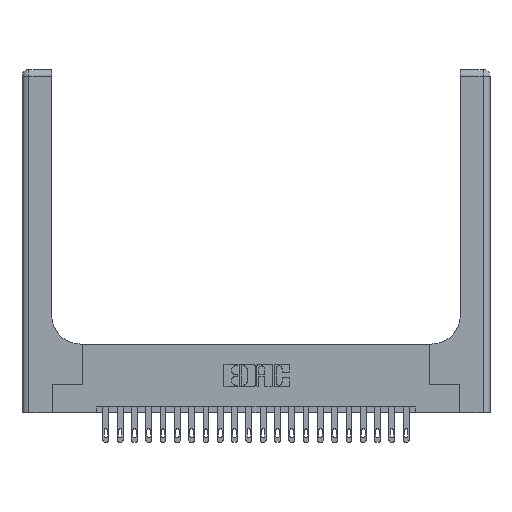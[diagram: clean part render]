
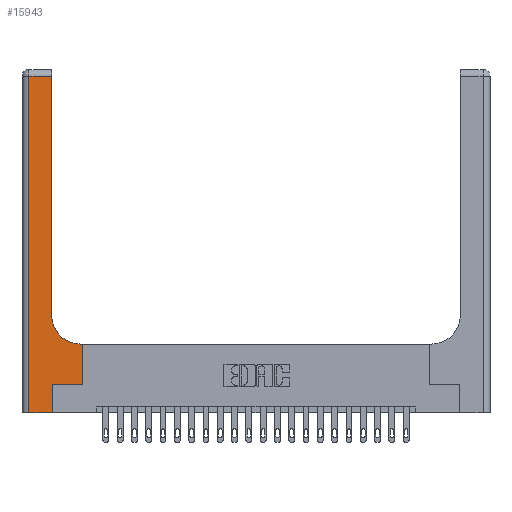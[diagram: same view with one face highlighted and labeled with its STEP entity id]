
A CAD part, top view. The second image highlights one B-rep face of the part: STEP entity #15943.
In plain terms, the highlighted planar face has unit normal (0, 0, 1).
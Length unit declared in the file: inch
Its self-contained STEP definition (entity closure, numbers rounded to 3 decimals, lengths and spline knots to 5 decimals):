
#837 = LINE ( 'NONE', #6121, #18668 ) ;
#1237 = LINE ( 'NONE', #21724, #15474 ) ;
#1333 = VERTEX_POINT ( 'NONE', #20239 ) ;
#1454 = CARTESIAN_POINT ( 'NONE',  ( 0.51, 0.6, 0.37 ) ) ;
#1460 = ORIENTED_EDGE ( 'NONE', *, *, #13298, .T. ) ;
#1658 = AXIS2_PLACEMENT_3D ( 'NONE', #1667, #21131, #7371 ) ;
#1667 = CARTESIAN_POINT ( 'NONE',  ( 0.51, 0.85, 0.37 ) ) ;
#2222 = LINE ( 'NONE', #19286, #21287 ) ;
#2387 = CARTESIAN_POINT ( 'NONE',  ( 0.06, 0., 0.37 ) ) ;
#2440 = DIRECTION ( 'NONE',  ( -1., 0., 0. ) ) ;
#2562 = DIRECTION ( 'NONE',  ( -1., 0., 0. ) ) ;
#3613 = DIRECTION ( 'NONE',  ( 0., 1., 0. ) ) ;
#3984 = ORIENTED_EDGE ( 'NONE', *, *, #19985, .T. ) ;
#4340 = EDGE_CURVE ( 'NONE', #7423, #19942, #9460, .T. ) ;
#4739 = EDGE_CURVE ( 'NONE', #1333, #20100, #837, .T. ) ;
#4877 = EDGE_CURVE ( 'NONE', #13815, #1333, #10093, .T. ) ;
#5120 = ORIENTED_EDGE ( 'NONE', *, *, #4877, .T. ) ;
#5781 = VECTOR ( 'NONE', #2562, 39.37008 ) ;
#6121 = CARTESIAN_POINT ( 'NONE',  ( 0.26, 0.6, 0.37 ) ) ;
#6176 = VERTEX_POINT ( 'NONE', #2387 ) ;
#6361 = ORIENTED_EDGE ( 'NONE', *, *, #13283, .T. ) ;
#6699 = CARTESIAN_POINT ( 'NONE',  ( 0.26, 2.94, 0.37 ) ) ;
#6926 = EDGE_CURVE ( 'NONE', #20100, #11942, #7878, .T. ) ;
#7192 = VERTEX_POINT ( 'NONE', #6699 ) ;
#7371 = DIRECTION ( 'NONE',  ( 1., 0., 0. ) ) ;
#7423 = VERTEX_POINT ( 'NONE', #18106 ) ;
#7878 = CIRCLE ( 'NONE', #1658, 0.25 ) ;
#8393 = VECTOR ( 'NONE', #16420, 39.37008 ) ;
#8433 = EDGE_LOOP ( 'NONE', ( #14188, #6361, #1460, #10906, #18893, #3984, #5120, #10993, #22576 ) ) ;
#9196 = AXIS2_PLACEMENT_3D ( 'NONE', #15601, #13441, #22366 ) ;
#9460 = LINE ( 'NONE', #11390, #8393 ) ;
#10093 = LINE ( 'NONE', #16956, #21581 ) ;
#10315 = DIRECTION ( 'NONE',  ( 0., 1., 0. ) ) ;
#10647 = EDGE_CURVE ( 'NONE', #6176, #7423, #16648, .T. ) ;
#10906 = ORIENTED_EDGE ( 'NONE', *, *, #10647, .T. ) ;
#10993 = ORIENTED_EDGE ( 'NONE', *, *, #4739, .T. ) ;
#11020 = LINE ( 'NONE', #16397, #12312 ) ;
#11390 = CARTESIAN_POINT ( 'NONE',  ( 0.265, 0., 0.37 ) ) ;
#11942 = VERTEX_POINT ( 'NONE', #13566 ) ;
#12312 = VECTOR ( 'NONE', #16170, 39.37008 ) ;
#12857 = CARTESIAN_POINT ( 'NONE',  ( 0., 0., 0.37 ) ) ;
#12948 = LINE ( 'NONE', #14680, #5781 ) ;
#13283 = EDGE_CURVE ( 'NONE', #7192, #22095, #12948, .T. ) ;
#13298 = EDGE_CURVE ( 'NONE', #22095, #6176, #11020, .T. ) ;
#13441 = DIRECTION ( 'NONE',  ( 0., 0., -1. ) ) ;
#13566 = CARTESIAN_POINT ( 'NONE',  ( 0.26, 0.85, 0.37 ) ) ;
#13815 = VERTEX_POINT ( 'NONE', #18553 ) ;
#14188 = ORIENTED_EDGE ( 'NONE', *, *, #16094, .T. ) ;
#14384 = CARTESIAN_POINT ( 'NONE',  ( 0.06, 2.94, 0.37 ) ) ;
#14680 = CARTESIAN_POINT ( 'NONE',  ( 0., 2.94, 0.37 ) ) ;
#15061 = DIRECTION ( 'NONE',  ( 1., 0., 0. ) ) ;
#15474 = VECTOR ( 'NONE', #15061, 39.37008 ) ;
#15601 = CARTESIAN_POINT ( 'NONE',  ( 0., 3., 0.37 ) ) ;
#15943 = ADVANCED_FACE ( 'NONE', ( #22256 ), #20567, .F. ) ;
#16094 = EDGE_CURVE ( 'NONE', #11942, #7192, #2222, .T. ) ;
#16170 = DIRECTION ( 'NONE',  ( 0., -1., 0. ) ) ;
#16397 = CARTESIAN_POINT ( 'NONE',  ( 0.06, 3., 0.37 ) ) ;
#16420 = DIRECTION ( 'NONE',  ( 0., 1., 0. ) ) ;
#16648 = LINE ( 'NONE', #12857, #17115 ) ;
#16956 = CARTESIAN_POINT ( 'NONE',  ( 0.528, 0.25, 0.37 ) ) ;
#17115 = VECTOR ( 'NONE', #18492, 39.37008 ) ;
#18106 = CARTESIAN_POINT ( 'NONE',  ( 0.265, 0., 0.37 ) ) ;
#18492 = DIRECTION ( 'NONE',  ( 1., 0., 0. ) ) ;
#18553 = CARTESIAN_POINT ( 'NONE',  ( 0.528, 0.25, 0.37 ) ) ;
#18668 = VECTOR ( 'NONE', #2440, 39.37008 ) ;
#18893 = ORIENTED_EDGE ( 'NONE', *, *, #4340, .T. ) ;
#19286 = CARTESIAN_POINT ( 'NONE',  ( 0.26, 3., 0.37 ) ) ;
#19942 = VERTEX_POINT ( 'NONE', #20027 ) ;
#19985 = EDGE_CURVE ( 'NONE', #19942, #13815, #1237, .T. ) ;
#20027 = CARTESIAN_POINT ( 'NONE',  ( 0.265, 0.25, 0.37 ) ) ;
#20100 = VERTEX_POINT ( 'NONE', #1454 ) ;
#20239 = CARTESIAN_POINT ( 'NONE',  ( 0.528, 0.6, 0.37 ) ) ;
#20567 = PLANE ( 'NONE',  #9196 ) ;
#21131 = DIRECTION ( 'NONE',  ( 0., 0., -1. ) ) ;
#21287 = VECTOR ( 'NONE', #3613, 39.37008 ) ;
#21581 = VECTOR ( 'NONE', #10315, 39.37008 ) ;
#21724 = CARTESIAN_POINT ( 'NONE',  ( 0.265, 0.25, 0.37 ) ) ;
#22095 = VERTEX_POINT ( 'NONE', #14384 ) ;
#22256 = FACE_OUTER_BOUND ( 'NONE', #8433, .T. ) ;
#22366 = DIRECTION ( 'NONE',  ( -1., 0., 0. ) ) ;
#22576 = ORIENTED_EDGE ( 'NONE', *, *, #6926, .T. ) ;
